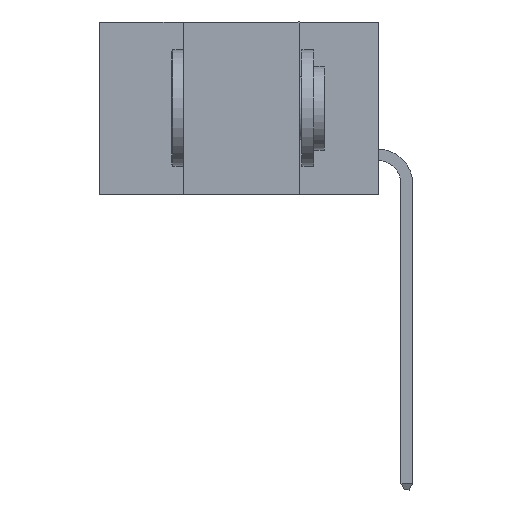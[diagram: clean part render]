
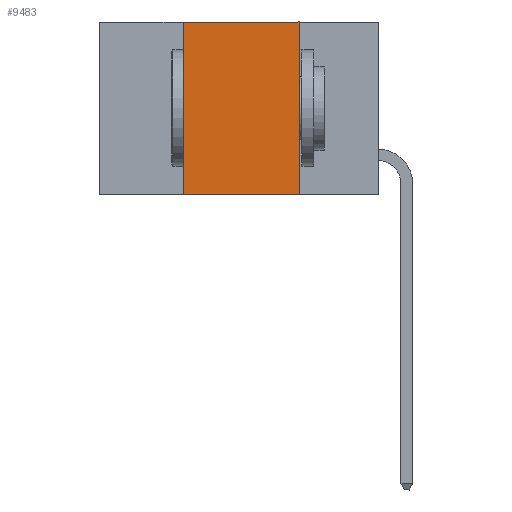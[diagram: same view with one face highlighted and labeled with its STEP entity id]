
A CAD part, left-side view. The second image highlights one B-rep face of the part: STEP entity #9483.
In plain terms, the highlighted planar face has unit normal (-1, 0, 0).
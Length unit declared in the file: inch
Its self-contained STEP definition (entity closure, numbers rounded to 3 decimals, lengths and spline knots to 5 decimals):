
#254 = EDGE_CURVE ( 'NONE', #4172, #6238, #1366, .T. ) ;
#652 = LINE ( 'NONE', #2547, #9637 ) ;
#1329 = EDGE_CURVE ( 'NONE', #4172, #4455, #2115, .T. ) ;
#1357 = DIRECTION ( 'NONE',  ( 0., -1., 0. ) ) ;
#1366 = LINE ( 'NONE', #1423, #3543 ) ;
#1410 = CARTESIAN_POINT ( 'NONE',  ( 0., 0.6, 0. ) ) ;
#1423 = CARTESIAN_POINT ( 'NONE',  ( 0., 0.42, -0.37 ) ) ;
#1939 = ORIENTED_EDGE ( 'NONE', *, *, #9133, .F. ) ;
#2115 = LINE ( 'NONE', #11069, #10518 ) ;
#2305 = DIRECTION ( 'NONE',  ( 1., 0., 0. ) ) ;
#2547 = CARTESIAN_POINT ( 'NONE',  ( 0., 0.17, -0.37 ) ) ;
#2686 = CARTESIAN_POINT ( 'NONE',  ( 0., 0.42, 0. ) ) ;
#3543 = VECTOR ( 'NONE', #10371, 39.37008 ) ;
#3836 = ORIENTED_EDGE ( 'NONE', *, *, #254, .F. ) ;
#3849 = CARTESIAN_POINT ( 'NONE',  ( 0., 0.42, -0.37 ) ) ;
#4090 = CARTESIAN_POINT ( 'NONE',  ( 0., 0.6, 0. ) ) ;
#4172 = VERTEX_POINT ( 'NONE', #3849 ) ;
#4455 = VERTEX_POINT ( 'NONE', #8951 ) ;
#4680 = VERTEX_POINT ( 'NONE', #9298 ) ;
#4972 = AXIS2_PLACEMENT_3D ( 'NONE', #4090, #2305, #7724 ) ;
#5096 = PLANE ( 'NONE',  #4972 ) ;
#5203 = EDGE_LOOP ( 'NONE', ( #1939, #10744, #3836, #5724 ) ) ;
#5506 = EDGE_CURVE ( 'NONE', #6238, #4680, #11294, .T. ) ;
#5724 = ORIENTED_EDGE ( 'NONE', *, *, #1329, .T. ) ;
#6238 = VERTEX_POINT ( 'NONE', #2686 ) ;
#6852 = DIRECTION ( 'NONE',  ( 0., -1., 0. ) ) ;
#6855 = FACE_OUTER_BOUND ( 'NONE', #5203, .T. ) ;
#7724 = DIRECTION ( 'NONE',  ( 0., 0., -1. ) ) ;
#8288 = VECTOR ( 'NONE', #6852, 39.37008 ) ;
#8844 = DIRECTION ( 'NONE',  ( 0., 0., -1. ) ) ;
#8951 = CARTESIAN_POINT ( 'NONE',  ( 0., 0.17, -0.37 ) ) ;
#9133 = EDGE_CURVE ( 'NONE', #4680, #4455, #652, .T. ) ;
#9298 = CARTESIAN_POINT ( 'NONE',  ( 0., 0.17, 0. ) ) ;
#9483 = ADVANCED_FACE ( 'NONE', ( #6855 ), #5096, .F. ) ;
#9637 = VECTOR ( 'NONE', #8844, 39.37008 ) ;
#10371 = DIRECTION ( 'NONE',  ( 0., 0., 1. ) ) ;
#10518 = VECTOR ( 'NONE', #1357, 39.37008 ) ;
#10744 = ORIENTED_EDGE ( 'NONE', *, *, #5506, .F. ) ;
#11069 = CARTESIAN_POINT ( 'NONE',  ( 0., 0.6, -0.37 ) ) ;
#11294 = LINE ( 'NONE', #1410, #8288 ) ;
